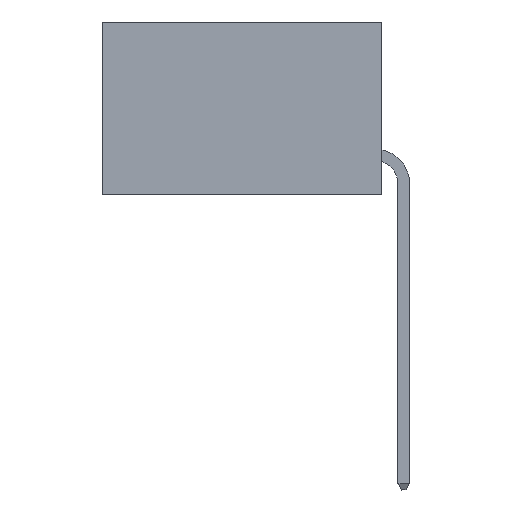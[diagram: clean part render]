
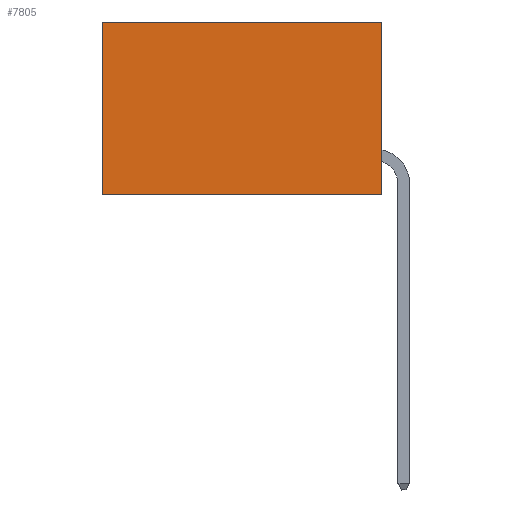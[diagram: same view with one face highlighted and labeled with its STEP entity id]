
A CAD part, left-side view. The second image highlights one B-rep face of the part: STEP entity #7805.
In plain terms, the highlighted planar face has unit normal (-1, 0, 0).
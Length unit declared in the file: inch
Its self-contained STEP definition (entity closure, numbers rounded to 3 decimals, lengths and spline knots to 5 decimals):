
#49 = VECTOR ( 'NONE', #4224, 39.37008 ) ;
#51 = DIRECTION ( 'NONE',  ( 0., 0., -1. ) ) ;
#208 = CARTESIAN_POINT ( 'NONE',  ( 0.2875, 0., -0.37 ) ) ;
#235 = VERTEX_POINT ( 'NONE', #2941 ) ;
#388 = DIRECTION ( 'NONE',  ( 1., 0., 0. ) ) ;
#1268 = CARTESIAN_POINT ( 'NONE',  ( 0.2875, 0.6, 0. ) ) ;
#1351 = ORIENTED_EDGE ( 'NONE', *, *, #1664, .F. ) ;
#1638 = VECTOR ( 'NONE', #3009, 39.37008 ) ;
#1664 = EDGE_CURVE ( 'NONE', #3156, #6465, #5174, .T. ) ;
#1756 = VECTOR ( 'NONE', #3329, 39.37008 ) ;
#2061 = AXIS2_PLACEMENT_3D ( 'NONE', #7790, #388, #51 ) ;
#2627 = VECTOR ( 'NONE', #2916, 39.37008 ) ;
#2764 = CARTESIAN_POINT ( 'NONE',  ( 0.2875, 0., 0. ) ) ;
#2916 = DIRECTION ( 'NONE',  ( 0., 1., 0. ) ) ;
#2926 = ORIENTED_EDGE ( 'NONE', *, *, #8648, .T. ) ;
#2941 = CARTESIAN_POINT ( 'NONE',  ( 0.2875, 0.6, -0.37 ) ) ;
#3009 = DIRECTION ( 'NONE',  ( 0., 1., 0. ) ) ;
#3156 = VERTEX_POINT ( 'NONE', #3201 ) ;
#3201 = CARTESIAN_POINT ( 'NONE',  ( 0.2875, 0., 0. ) ) ;
#3292 = LINE ( 'NONE', #7231, #2627 ) ;
#3329 = DIRECTION ( 'NONE',  ( 0., 0., -1. ) ) ;
#3486 = PLANE ( 'NONE',  #2061 ) ;
#3653 = LINE ( 'NONE', #8198, #1756 ) ;
#3772 = CARTESIAN_POINT ( 'NONE',  ( 0.2875, 0., -0.37 ) ) ;
#4224 = DIRECTION ( 'NONE',  ( 0., 0., -1. ) ) ;
#4470 = EDGE_CURVE ( 'NONE', #6465, #235, #5427, .T. ) ;
#4595 = ORIENTED_EDGE ( 'NONE', *, *, #4470, .F. ) ;
#5073 = EDGE_CURVE ( 'NONE', #3156, #5616, #3292, .T. ) ;
#5174 = LINE ( 'NONE', #2764, #49 ) ;
#5427 = LINE ( 'NONE', #3772, #1638 ) ;
#5616 = VERTEX_POINT ( 'NONE', #1268 ) ;
#5911 = FACE_OUTER_BOUND ( 'NONE', #6337, .T. ) ;
#6337 = EDGE_LOOP ( 'NONE', ( #2926, #4595, #1351, #9099 ) ) ;
#6465 = VERTEX_POINT ( 'NONE', #208 ) ;
#7231 = CARTESIAN_POINT ( 'NONE',  ( 0.2875, 0., 0. ) ) ;
#7790 = CARTESIAN_POINT ( 'NONE',  ( 0.2875, 0., 0. ) ) ;
#7805 = ADVANCED_FACE ( 'NONE', ( #5911 ), #3486, .F. ) ;
#8198 = CARTESIAN_POINT ( 'NONE',  ( 0.2875, 0.6, 0. ) ) ;
#8648 = EDGE_CURVE ( 'NONE', #5616, #235, #3653, .T. ) ;
#9099 = ORIENTED_EDGE ( 'NONE', *, *, #5073, .T. ) ;
